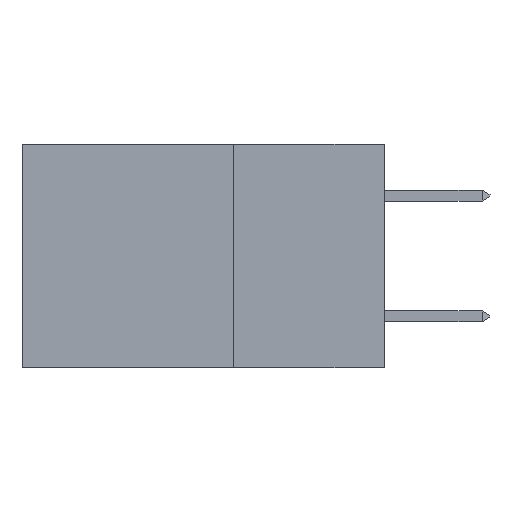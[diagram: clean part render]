
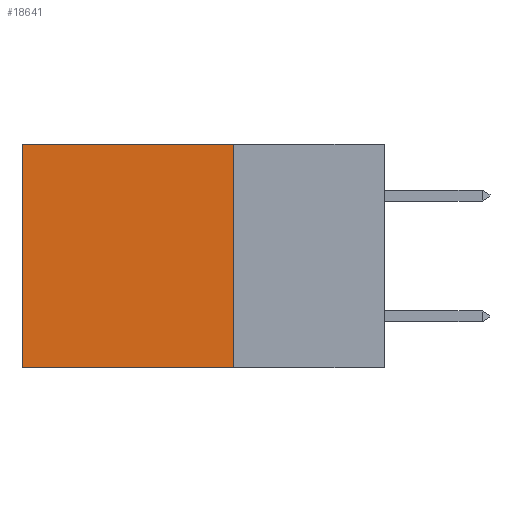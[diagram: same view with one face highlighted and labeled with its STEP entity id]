
A CAD part, left-side view. The second image highlights one B-rep face of the part: STEP entity #18641.
In plain terms, the highlighted planar face has unit normal (-1, 0, 0).
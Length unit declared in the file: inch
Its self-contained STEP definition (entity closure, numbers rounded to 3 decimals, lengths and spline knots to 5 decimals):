
#634 = ORIENTED_EDGE ( 'NONE', *, *, #18246, .T. ) ;
#718 = CARTESIAN_POINT ( 'NONE',  ( 0.2875, 0.25, 0. ) ) ;
#2627 = FACE_OUTER_BOUND ( 'NONE', #20586, .T. ) ;
#3578 = LINE ( 'NONE', #19268, #7931 ) ;
#5315 = CARTESIAN_POINT ( 'NONE',  ( 0.2875, 0.25, 0. ) ) ;
#5570 = VERTEX_POINT ( 'NONE', #14628 ) ;
#5791 = VERTEX_POINT ( 'NONE', #18740 ) ;
#7466 = CARTESIAN_POINT ( 'NONE',  ( 0.2875, 0.25, -0.37 ) ) ;
#7931 = VECTOR ( 'NONE', #10537, 39.37008 ) ;
#8064 = PLANE ( 'NONE',  #11283 ) ;
#8430 = ORIENTED_EDGE ( 'NONE', *, *, #13569, .F. ) ;
#8963 = LINE ( 'NONE', #13332, #21905 ) ;
#9078 = VECTOR ( 'NONE', #16355, 39.37008 ) ;
#9670 = LINE ( 'NONE', #7466, #9078 ) ;
#9953 = DIRECTION ( 'NONE',  ( 0., 0., -1. ) ) ;
#10028 = DIRECTION ( 'NONE',  ( 0., 1., 0. ) ) ;
#10537 = DIRECTION ( 'NONE',  ( 0., 0., -1. ) ) ;
#11283 = AXIS2_PLACEMENT_3D ( 'NONE', #15244, #20481, #9953 ) ;
#12341 = LINE ( 'NONE', #718, #15928 ) ;
#13062 = ORIENTED_EDGE ( 'NONE', *, *, #17316, .F. ) ;
#13332 = CARTESIAN_POINT ( 'NONE',  ( 0.2875, 0.25, 0. ) ) ;
#13569 = EDGE_CURVE ( 'NONE', #16568, #5570, #8963, .T. ) ;
#13621 = ORIENTED_EDGE ( 'NONE', *, *, #18684, .T. ) ;
#14628 = CARTESIAN_POINT ( 'NONE',  ( 0.2875, 0.25, -0.37 ) ) ;
#14739 = VERTEX_POINT ( 'NONE', #23191 ) ;
#15111 = DIRECTION ( 'NONE',  ( 0., 0., -1. ) ) ;
#15244 = CARTESIAN_POINT ( 'NONE',  ( 0.2875, 0.25, 0. ) ) ;
#15928 = VECTOR ( 'NONE', #10028, 39.37008 ) ;
#16355 = DIRECTION ( 'NONE',  ( 0., 1., 0. ) ) ;
#16568 = VERTEX_POINT ( 'NONE', #5315 ) ;
#17316 = EDGE_CURVE ( 'NONE', #5570, #5791, #9670, .T. ) ;
#18246 = EDGE_CURVE ( 'NONE', #14739, #5791, #3578, .T. ) ;
#18641 = ADVANCED_FACE ( 'NONE', ( #2627 ), #8064, .F. ) ;
#18684 = EDGE_CURVE ( 'NONE', #16568, #14739, #12341, .T. ) ;
#18740 = CARTESIAN_POINT ( 'NONE',  ( 0.2875, 0.6, -0.37 ) ) ;
#19268 = CARTESIAN_POINT ( 'NONE',  ( 0.2875, 0.6, 0. ) ) ;
#20481 = DIRECTION ( 'NONE',  ( 1., 0., 0. ) ) ;
#20586 = EDGE_LOOP ( 'NONE', ( #634, #13062, #8430, #13621 ) ) ;
#21905 = VECTOR ( 'NONE', #15111, 39.37008 ) ;
#23191 = CARTESIAN_POINT ( 'NONE',  ( 0.2875, 0.6, 0. ) ) ;
